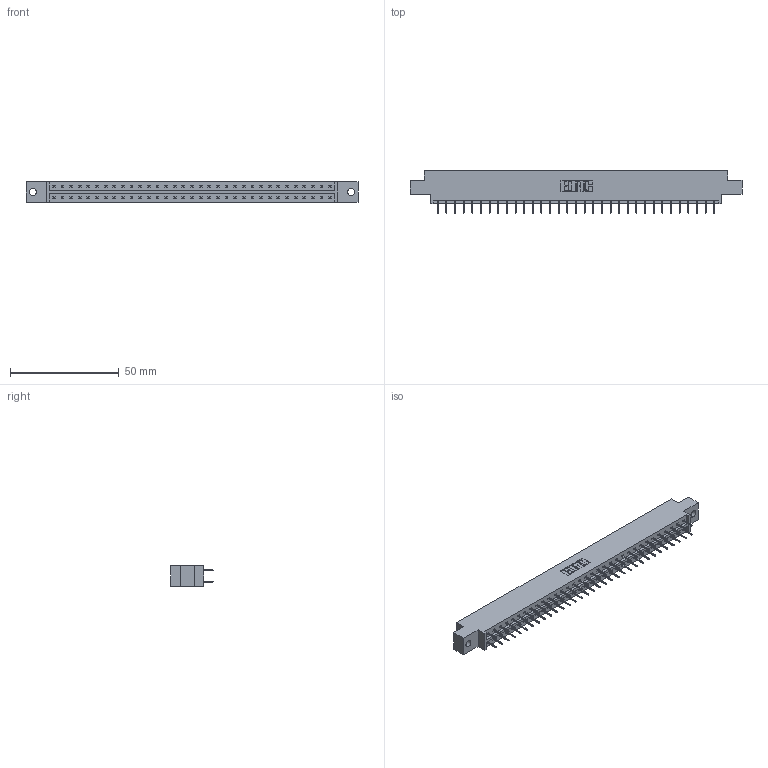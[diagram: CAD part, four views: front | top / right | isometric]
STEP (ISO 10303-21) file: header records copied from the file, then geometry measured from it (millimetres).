
FILE_DESCRIPTION (( 'STEP AP203' ), '1' );
FILE_NAME ('833-066-524-802.STEP', '2020-06-05T08:45:50', ( '' ), ( '' ), 'SwSTEP 2.0', 'SolidWorks 2020', '' );
FILE_SCHEMA (( 'CONFIG_CONTROL_DESIGN' ));
Length unit declared in the file: inch
Products named in the file (3): 833-066-524-802; 833 Part_Offset - .128 Dia; 345-292-001_345-293-124
Assembly tree (67 placements, depth 2):
  833-066-524-802
    833 Part_Offset - .128 Dia
    345-292-001_345-293-124  x66
Bounding box: 152.3 x 19.69 x 9.4 mm (x, y, z)
Volume: 15100.3 mm3; surface area: 17403.3 mm2
Topology: 67 solids, 67 shells, 3814 faces, 10817 edges, 6946 vertices
Faces by surface type: plane 2846, cylinder 968
Entity records: 22603 total; most frequent: CARTESIAN_POINT 3758, ORIENTED_EDGE 3694, DIRECTION 3227, EDGE_CURVE 1847, VECTOR 1723, LINE 1723, VERTEX_POINT 1226, AXIS2_PLACEMENT_3D 752
